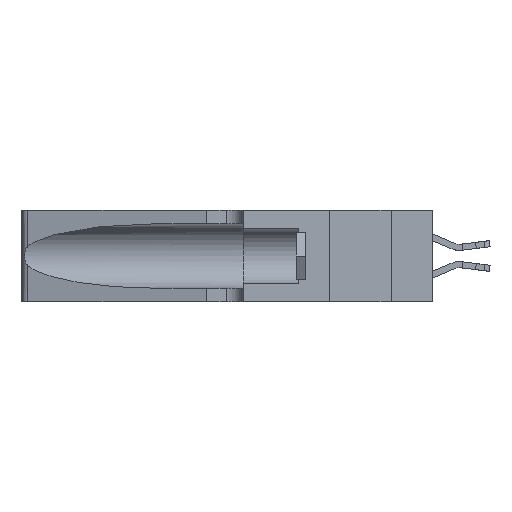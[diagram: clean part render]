
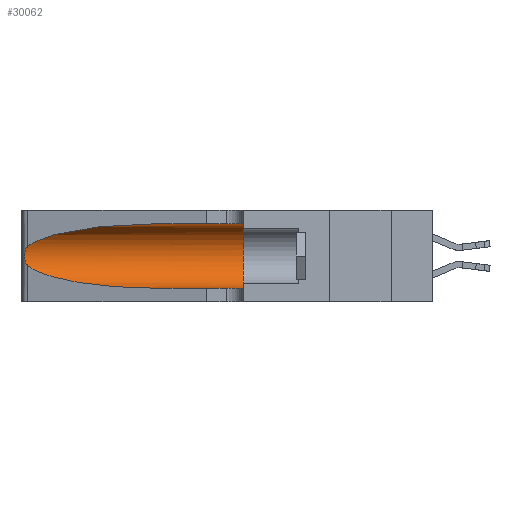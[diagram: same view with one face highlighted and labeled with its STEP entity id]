
A CAD part, left-side view. The second image highlights one B-rep face of the part: STEP entity #30062.
In plain terms, the highlighted cylindrical face has radius 3.308 mm (diameter 6.617 mm), a partial arc.
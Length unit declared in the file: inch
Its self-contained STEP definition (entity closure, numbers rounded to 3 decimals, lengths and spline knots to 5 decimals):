
#668 = ORIENTED_EDGE ( 'NONE', *, *, #9048, .T. ) ;
#737 = EDGE_CURVE ( 'NONE', #28741, #7766, #5350, .T. ) ;
#1038 = CARTESIAN_POINT ( 'NONE',  ( 0.1305, 1.61858, 0.31525 ) ) ;
#1059 = LINE ( 'NONE', #1038, #30688 ) ;
#2033 = CARTESIAN_POINT ( 'NONE',  ( 0.18966, 0.96281, 0.31525 ) ) ;
#2132 = CARTESIAN_POINT ( 'NONE',  ( 0.1305, 0.72297, 0.31525 ) ) ;
#2875 = CARTESIAN_POINT ( 'NONE',  ( 0.25487, 1.22718, 0.14631 ) ) ;
#3715 = CARTESIAN_POINT ( 'NONE',  ( 0.25789, 1.23486, 0.15765 ) ) ;
#4650 = CARTESIAN_POINT ( 'NONE',  ( 0.2373, 1.15595, 0.28018 ) ) ;
#4740 = DIRECTION ( 'NONE',  ( 0., 1., 0. ) ) ;
#5187 = CARTESIAN_POINT ( 'NONE',  ( 0.26017, 1.23833, 0.17102 ) ) ;
#5350 = LINE ( 'NONE', #8953, #22219 ) ;
#6285 = VERTEX_POINT ( 'NONE', #7607 ) ;
#6361 = ORIENTED_EDGE ( 'NONE', *, *, #13490, .T. ) ;
#6615 = EDGE_CURVE ( 'NONE', #25067, #11529, #1059, .T. ) ;
#7607 = CARTESIAN_POINT ( 'NONE',  ( 0.25487, 1.22718, 0.22369 ) ) ;
#7624 = CARTESIAN_POINT ( 'NONE',  ( 0.25555, 1.22993, 0.14849 ) ) ;
#7766 = VERTEX_POINT ( 'NONE', #27100 ) ;
#8430 = CARTESIAN_POINT ( 'NONE',  ( 0.2373, 1.15595, 0.08982 ) ) ;
#8691 = DIRECTION ( 'NONE',  ( 0., -1., 0. ) ) ;
#8953 = CARTESIAN_POINT ( 'NONE',  ( 0.1305, 1.61858, 0.05475 ) ) ;
#9048 = EDGE_CURVE ( 'NONE', #6285, #28755, #23731, .T. ) ;
#9188 = ORIENTED_EDGE ( 'NONE', *, *, #26262, .F. ) ;
#9244 = EDGE_CURVE ( 'NONE', #28755, #28741, #27035, .T. ) ;
#9417 = ORIENTED_EDGE ( 'NONE', *, *, #6615, .F. ) ;
#9500 = CARTESIAN_POINT ( 'NONE',  ( 0.25487, 1.22718, 0.22369 ) ) ;
#9725 = CARTESIAN_POINT ( 'NONE',  ( 0.25787, 1.23484, 0.2124 ) ) ;
#10055 = CIRCLE ( 'NONE', #11494, 0.13025 ) ;
#10234 = CARTESIAN_POINT ( 'NONE',  ( 0.26075, 1.23896, 0.19203 ) ) ;
#10342 = CARTESIAN_POINT ( 'NONE',  ( 0.25856, 1.23593, 0.16098 ) ) ;
#11075 = CARTESIAN_POINT ( 'NONE',  ( 0.18966, 0.96281, 0.05475 ) ) ;
#11111 = ORIENTED_EDGE ( 'NONE', *, *, #9244, .T. ) ;
#11494 = AXIS2_PLACEMENT_3D ( 'NONE', #26236, #4740, #18283 ) ;
#11529 = VERTEX_POINT ( 'NONE', #20723 ) ;
#12058 = CARTESIAN_POINT ( 'NONE',  ( 0.25555, 1.22994, 0.2215 ) ) ;
#12160 = CARTESIAN_POINT ( 'NONE',  ( 0.25487, 1.22718, 0.22369 ) ) ;
#13428 = CARTESIAN_POINT ( 'NONE',  ( 0.1305, 1.61858, 0.185 ) ) ;
#13490 = EDGE_CURVE ( 'NONE', #25067, #6285, #16703, .T. ) ;
#13501 = DIRECTION ( 'NONE',  ( 0., -1., 0. ) ) ;
#15679 = ORIENTED_EDGE ( 'NONE', *, *, #737, .T. ) ;
#16703 =( BOUNDED_CURVE ( )  B_SPLINE_CURVE ( 3, ( #2132, #2033, #4650, #9500 ),
 .UNSPECIFIED., .F., .T. ) 
 B_SPLINE_CURVE_WITH_KNOTS ( ( 4, 4 ),
 ( 1.5708, 2.84003 ),
 .UNSPECIFIED. ) 
 CURVE ( )  GEOMETRIC_REPRESENTATION_ITEM ( )  RATIONAL_B_SPLINE_CURVE ( ( 1., 0.87, 0.87, 1. ) ) 
 REPRESENTATION_ITEM ( '' )  );
#16763 = AXIS2_PLACEMENT_3D ( 'NONE', #13428, #8691, #23119 ) ;
#17266 = CARTESIAN_POINT ( 'NONE',  ( 0.26018, 1.23835, 0.19895 ) ) ;
#18283 = DIRECTION ( 'NONE',  ( 0., 0., 1. ) ) ;
#18294 = CYLINDRICAL_SURFACE ( 'NONE', #16763, 0.13025 ) ;
#18839 = CARTESIAN_POINT ( 'NONE',  ( 0.1305, 0.72297, 0.31525 ) ) ;
#19257 = CARTESIAN_POINT ( 'NONE',  ( 0.25639, 1.23184, 0.21858 ) ) ;
#19759 = CARTESIAN_POINT ( 'NONE',  ( 0.25639, 1.23186, 0.15144 ) ) ;
#20723 = CARTESIAN_POINT ( 'NONE',  ( 0.1305, 0.35, 0.31525 ) ) ;
#22219 = VECTOR ( 'NONE', #13501, 39.37008 ) ;
#22754 = CARTESIAN_POINT ( 'NONE',  ( 0.25487, 1.22718, 0.14631 ) ) ;
#23119 = DIRECTION ( 'NONE',  ( 0., 0., -1. ) ) ;
#23731 = B_SPLINE_CURVE_WITH_KNOTS ( 'NONE', 3,
 ( #12160, #12058, #19257, #9725, #24148, #17266, #10234, #29509, #5187, #10342, #3715, #19759, #7624, #2875 ),
 .UNSPECIFIED., .F., .F.,
 ( 4, 2, 2, 2, 2, 2, 4 ),
 ( 0., 0.00027, 0.00053, 0.00107, 0.0016, 0.00187, 0.00214 ),
 .UNSPECIFIED. ) ;
#24104 = CARTESIAN_POINT ( 'NONE',  ( 0.1305, 0.72297, 0.05475 ) ) ;
#24148 = CARTESIAN_POINT ( 'NONE',  ( 0.25854, 1.2359, 0.20912 ) ) ;
#24629 = EDGE_LOOP ( 'NONE', ( #6361, #668, #11111, #15679, #9188, #9417 ) ) ;
#25067 = VERTEX_POINT ( 'NONE', #18839 ) ;
#25155 = CARTESIAN_POINT ( 'NONE',  ( 0.1305, 0.72297, 0.05475 ) ) ;
#25320 = DIRECTION ( 'NONE',  ( 0., -1., 0. ) ) ;
#25367 = CARTESIAN_POINT ( 'NONE',  ( 0.25487, 1.22718, 0.14631 ) ) ;
#26236 = CARTESIAN_POINT ( 'NONE',  ( 0.1305, 0.35, 0.185 ) ) ;
#26262 = EDGE_CURVE ( 'NONE', #11529, #7766, #10055, .T. ) ;
#27035 =( BOUNDED_CURVE ( )  B_SPLINE_CURVE ( 3, ( #22754, #8430, #11075, #25155 ),
 .UNSPECIFIED., .F., .T. ) 
 B_SPLINE_CURVE_WITH_KNOTS ( ( 4, 4 ),
 ( 3.44316, 4.71239 ),
 .UNSPECIFIED. ) 
 CURVE ( )  GEOMETRIC_REPRESENTATION_ITEM ( )  RATIONAL_B_SPLINE_CURVE ( ( 1., 0.87, 0.87, 1. ) ) 
 REPRESENTATION_ITEM ( '' )  );
#27100 = CARTESIAN_POINT ( 'NONE',  ( 0.1305, 0.35, 0.05475 ) ) ;
#28741 = VERTEX_POINT ( 'NONE', #24104 ) ;
#28755 = VERTEX_POINT ( 'NONE', #25367 ) ;
#29509 = CARTESIAN_POINT ( 'NONE',  ( 0.26075, 1.23896, 0.178 ) ) ;
#30062 = ADVANCED_FACE ( 'NONE', ( #30310 ), #18294, .F. ) ;
#30310 = FACE_OUTER_BOUND ( 'NONE', #24629, .T. ) ;
#30688 = VECTOR ( 'NONE', #25320, 39.37008 ) ;
